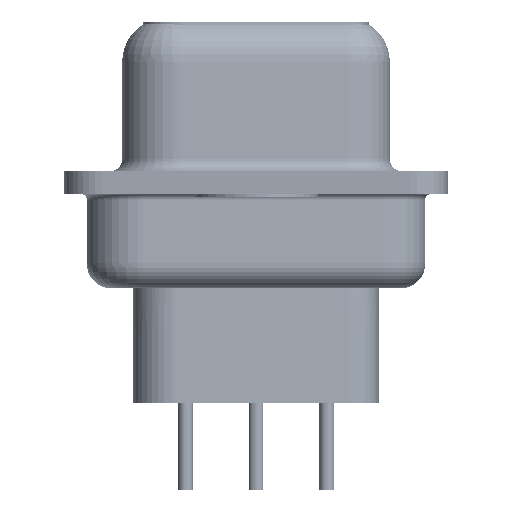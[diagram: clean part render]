
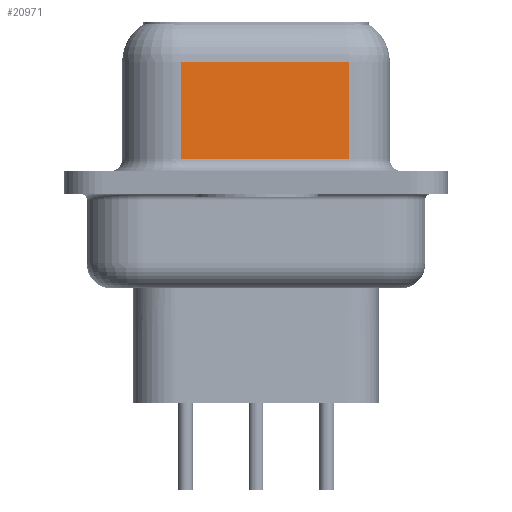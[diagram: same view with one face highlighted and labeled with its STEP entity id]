
A CAD part, left-side view. The second image highlights one B-rep face of the part: STEP entity #20971.
In plain terms, the highlighted planar face has unit normal (-0.985, -0.174, 0).
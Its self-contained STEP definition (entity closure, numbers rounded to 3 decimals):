
#225 = ORIENTED_EDGE ( 'NONE', *, *, #13497, .T. ) ;
#1040 = EDGE_LOOP ( 'NONE', ( #38932, #225, #14210, #4197 ) ) ;
#3961 = VERTEX_POINT ( 'NONE', #22819 ) ;
#4197 = ORIENTED_EDGE ( 'NONE', *, *, #42497, .T. ) ;
#6070 = DIRECTION ( 'NONE',  ( 0., 0., -1. ) ) ;
#7291 = LINE ( 'NONE', #24639, #7909 ) ;
#7637 = DIRECTION ( 'NONE',  ( 0.985, 0.174, 0. ) ) ;
#7909 = VECTOR ( 'NONE', #27599, 1000. ) ;
#8137 = VERTEX_POINT ( 'NONE', #32726 ) ;
#11194 = LINE ( 'NONE', #42290, #28511 ) ;
#13497 = EDGE_CURVE ( 'NONE', #31546, #3961, #11194, .T. ) ;
#14210 = ORIENTED_EDGE ( 'NONE', *, *, #25687, .T. ) ;
#20971 = ADVANCED_FACE ( 'NONE', ( #38972 ), #31995, .F. ) ;
#21912 = CARTESIAN_POINT ( 'NONE',  ( 5.621, -3.722, 4.85 ) ) ;
#22109 = VECTOR ( 'NONE', #6070, 1000. ) ;
#22819 = CARTESIAN_POINT ( 'NONE',  ( 4.43, 3.028, 4.85 ) ) ;
#24316 = VERTEX_POINT ( 'NONE', #27681 ) ;
#24639 = CARTESIAN_POINT ( 'NONE',  ( 5.621, -3.722, 0.95 ) ) ;
#25687 = EDGE_CURVE ( 'NONE', #3961, #8137, #31792, .T. ) ;
#27599 = DIRECTION ( 'NONE',  ( 0.174, -0.985, 0. ) ) ;
#27681 = CARTESIAN_POINT ( 'NONE',  ( 5.621, -3.722, 0.95 ) ) ;
#28511 = VECTOR ( 'NONE', #35081, 1000. ) ;
#28618 = DIRECTION ( 'NONE',  ( -0.174, 0.985, 0. ) ) ;
#29282 = CARTESIAN_POINT ( 'NONE',  ( 4.43, 3.028, 6.6 ) ) ;
#29520 = DIRECTION ( 'NONE',  ( 0., 0., -1. ) ) ;
#31546 = VERTEX_POINT ( 'NONE', #21912 ) ;
#31792 = LINE ( 'NONE', #29282, #37782 ) ;
#31995 = PLANE ( 'NONE',  #32852 ) ;
#32726 = CARTESIAN_POINT ( 'NONE',  ( 4.43, 3.028, 0.95 ) ) ;
#32852 = AXIS2_PLACEMENT_3D ( 'NONE', #35372, #7637, #28618 ) ;
#34029 = CARTESIAN_POINT ( 'NONE',  ( 5.621, -3.722, 6.6 ) ) ;
#35081 = DIRECTION ( 'NONE',  ( -0.174, 0.985, 0. ) ) ;
#35372 = CARTESIAN_POINT ( 'NONE',  ( 5.621, -3.722, 6.6 ) ) ;
#37782 = VECTOR ( 'NONE', #29520, 1000. ) ;
#38932 = ORIENTED_EDGE ( 'NONE', *, *, #42676, .F. ) ;
#38972 = FACE_OUTER_BOUND ( 'NONE', #1040, .T. ) ;
#42290 = CARTESIAN_POINT ( 'NONE',  ( 5.621, -3.722, 4.85 ) ) ;
#42497 = EDGE_CURVE ( 'NONE', #8137, #24316, #7291, .T. ) ;
#42676 = EDGE_CURVE ( 'NONE', #31546, #24316, #43962, .T. ) ;
#43962 = LINE ( 'NONE', #34029, #22109 ) ;
